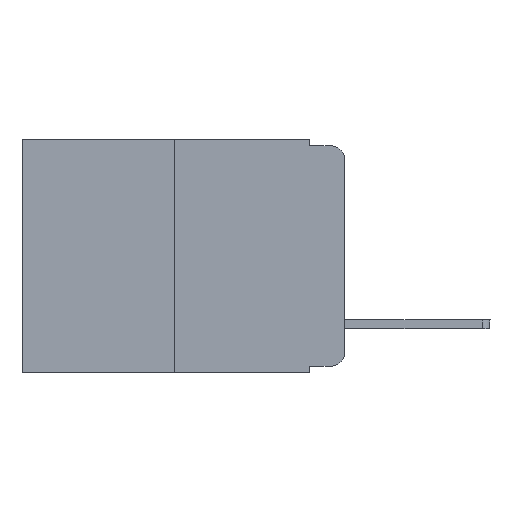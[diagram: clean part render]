
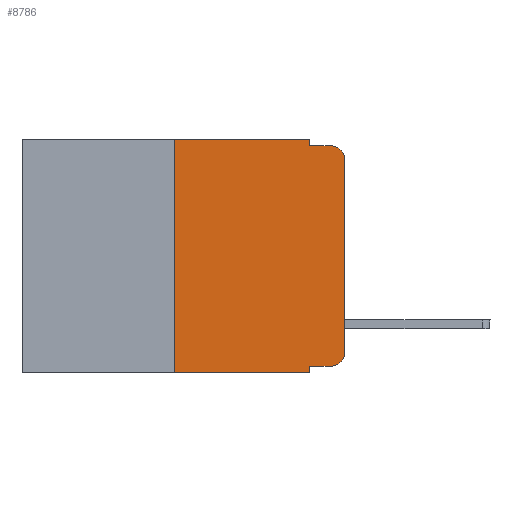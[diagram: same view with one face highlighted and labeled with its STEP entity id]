
A CAD part, left-side view. The second image highlights one B-rep face of the part: STEP entity #8786.
In plain terms, the highlighted planar face has unit normal (-1, 0, 0).
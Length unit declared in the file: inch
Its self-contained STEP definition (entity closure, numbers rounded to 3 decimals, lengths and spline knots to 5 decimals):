
#667 = EDGE_CURVE ( 'NONE', #10246, #11762, #2516, .T. ) ;
#1232 = LINE ( 'NONE', #14281, #9371 ) ;
#1288 = PLANE ( 'NONE',  #8417 ) ;
#1391 = DIRECTION ( 'NONE',  ( 0., -1., 0. ) ) ;
#1600 = DIRECTION ( 'NONE',  ( 1., 0., 0. ) ) ;
#1825 = CARTESIAN_POINT ( 'NONE',  ( 0., 0.02, -0.03 ) ) ;
#1990 = DIRECTION ( 'NONE',  ( -1., 0., 0. ) ) ;
#2516 = CIRCLE ( 'NONE', #4518, 0.02 ) ;
#2681 = CARTESIAN_POINT ( 'NONE',  ( 0., 0.051, 0. ) ) ;
#3585 = DIRECTION ( 'NONE',  ( 0., 0., 1. ) ) ;
#3679 = CIRCLE ( 'NONE', #5413, 0.02 ) ;
#3746 = VERTEX_POINT ( 'NONE', #10180 ) ;
#3747 = DIRECTION ( 'NONE',  ( 0., 0., 1. ) ) ;
#4075 = EDGE_CURVE ( 'NONE', #14331, #8205, #3679, .T. ) ;
#4138 = CARTESIAN_POINT ( 'NONE',  ( 0., 0.02, -0.313 ) ) ;
#4140 = DIRECTION ( 'NONE',  ( 0., -1., 0. ) ) ;
#4169 = ORIENTED_EDGE ( 'NONE', *, *, #4075, .T. ) ;
#4255 = DIRECTION ( 'NONE',  ( 0., 0., -1. ) ) ;
#4518 = AXIS2_PLACEMENT_3D ( 'NONE', #1825, #1990, #4255 ) ;
#5149 = EDGE_CURVE ( 'NONE', #12982, #13312, #11440, .T. ) ;
#5413 = AXIS2_PLACEMENT_3D ( 'NONE', #4138, #8889, #13507 ) ;
#5420 = DIRECTION ( 'NONE',  ( 0., -1., 0. ) ) ;
#5581 = ORIENTED_EDGE ( 'NONE', *, *, #12744, .F. ) ;
#5709 = VECTOR ( 'NONE', #13709, 39.37008 ) ;
#5800 = CARTESIAN_POINT ( 'NONE',  ( 0., 0., 0. ) ) ;
#6046 = EDGE_CURVE ( 'NONE', #3746, #7562, #14821, .T. ) ;
#6140 = FACE_OUTER_BOUND ( 'NONE', #13904, .T. ) ;
#6276 = DIRECTION ( 'NONE',  ( 0., 0., -1. ) ) ;
#6404 = ORIENTED_EDGE ( 'NONE', *, *, #10711, .F. ) ;
#6592 = LINE ( 'NONE', #8933, #5709 ) ;
#7273 = VECTOR ( 'NONE', #4140, 39.37008 ) ;
#7327 = CARTESIAN_POINT ( 'NONE',  ( 0., 0.051, -0.01 ) ) ;
#7517 = ORIENTED_EDGE ( 'NONE', *, *, #6046, .F. ) ;
#7562 = VERTEX_POINT ( 'NONE', #8498 ) ;
#7696 = VECTOR ( 'NONE', #3747, 39.37008 ) ;
#7961 = ORIENTED_EDGE ( 'NONE', *, *, #667, .T. ) ;
#8205 = VERTEX_POINT ( 'NONE', #11289 ) ;
#8236 = EDGE_CURVE ( 'NONE', #8439, #14331, #6592, .T. ) ;
#8250 = ORIENTED_EDGE ( 'NONE', *, *, #5149, .T. ) ;
#8417 = AXIS2_PLACEMENT_3D ( 'NONE', #14411, #1600, #13165 ) ;
#8439 = VERTEX_POINT ( 'NONE', #14473 ) ;
#8498 = CARTESIAN_POINT ( 'NONE',  ( 0., 0.051, 0. ) ) ;
#8533 = ORIENTED_EDGE ( 'NONE', *, *, #10507, .F. ) ;
#8554 = ORIENTED_EDGE ( 'NONE', *, *, #15274, .T. ) ;
#8786 = ADVANCED_FACE ( 'NONE', ( #6140 ), #1288, .F. ) ;
#8889 = DIRECTION ( 'NONE',  ( -1., 0., 0. ) ) ;
#8933 = CARTESIAN_POINT ( 'NONE',  ( 0., 0.051, -0.333 ) ) ;
#9371 = VECTOR ( 'NONE', #3585, 39.37008 ) ;
#9713 = EDGE_CURVE ( 'NONE', #11615, #11762, #13269, .T. ) ;
#9945 = LINE ( 'NONE', #2681, #12816 ) ;
#9957 = CARTESIAN_POINT ( 'NONE',  ( 0., 0.473, -0.343 ) ) ;
#10180 = CARTESIAN_POINT ( 'NONE',  ( 0., 0.25, 0. ) ) ;
#10246 = VERTEX_POINT ( 'NONE', #10262 ) ;
#10262 = CARTESIAN_POINT ( 'NONE',  ( 0., 0., -0.03 ) ) ;
#10319 = LINE ( 'NONE', #13847, #13097 ) ;
#10324 = VECTOR ( 'NONE', #1391, 39.37008 ) ;
#10367 = CARTESIAN_POINT ( 'NONE',  ( 0., 0.02, -0.333 ) ) ;
#10507 = EDGE_CURVE ( 'NONE', #7562, #11615, #9945, .T. ) ;
#10711 = EDGE_CURVE ( 'NONE', #8439, #13312, #10319, .T. ) ;
#11101 = CARTESIAN_POINT ( 'NONE',  ( 0., 0.473, 0. ) ) ;
#11289 = CARTESIAN_POINT ( 'NONE',  ( 0., 0., -0.313 ) ) ;
#11440 = LINE ( 'NONE', #9957, #11774 ) ;
#11615 = VERTEX_POINT ( 'NONE', #13009 ) ;
#11762 = VERTEX_POINT ( 'NONE', #13535 ) ;
#11774 = VECTOR ( 'NONE', #5420, 39.37008 ) ;
#12559 = CARTESIAN_POINT ( 'NONE',  ( 0., 0.25, -0.343 ) ) ;
#12744 = EDGE_CURVE ( 'NONE', #12982, #3746, #1232, .T. ) ;
#12816 = VECTOR ( 'NONE', #6276, 39.37008 ) ;
#12982 = VERTEX_POINT ( 'NONE', #12559 ) ;
#13009 = CARTESIAN_POINT ( 'NONE',  ( 0., 0.051, -0.01 ) ) ;
#13097 = VECTOR ( 'NONE', #13769, 39.37008 ) ;
#13165 = DIRECTION ( 'NONE',  ( 0., 0., -1. ) ) ;
#13269 = LINE ( 'NONE', #7327, #10324 ) ;
#13312 = VERTEX_POINT ( 'NONE', #14341 ) ;
#13507 = DIRECTION ( 'NONE',  ( 0., 0., -1. ) ) ;
#13535 = CARTESIAN_POINT ( 'NONE',  ( 0., 0.02, -0.01 ) ) ;
#13709 = DIRECTION ( 'NONE',  ( 0., -1., 0. ) ) ;
#13769 = DIRECTION ( 'NONE',  ( 0., 0., -1. ) ) ;
#13847 = CARTESIAN_POINT ( 'NONE',  ( 0., 0.051, 0. ) ) ;
#13904 = EDGE_LOOP ( 'NONE', ( #8554, #7961, #14890, #8533, #7517, #5581, #8250, #6404, #14441, #4169 ) ) ;
#14281 = CARTESIAN_POINT ( 'NONE',  ( 0., 0.25, 0. ) ) ;
#14331 = VERTEX_POINT ( 'NONE', #10367 ) ;
#14341 = CARTESIAN_POINT ( 'NONE',  ( 0., 0.051, -0.343 ) ) ;
#14411 = CARTESIAN_POINT ( 'NONE',  ( 0., 0.473, 0. ) ) ;
#14441 = ORIENTED_EDGE ( 'NONE', *, *, #8236, .T. ) ;
#14442 = LINE ( 'NONE', #5800, #7696 ) ;
#14473 = CARTESIAN_POINT ( 'NONE',  ( 0., 0.051, -0.333 ) ) ;
#14821 = LINE ( 'NONE', #11101, #7273 ) ;
#14890 = ORIENTED_EDGE ( 'NONE', *, *, #9713, .F. ) ;
#15274 = EDGE_CURVE ( 'NONE', #8205, #10246, #14442, .T. ) ;
